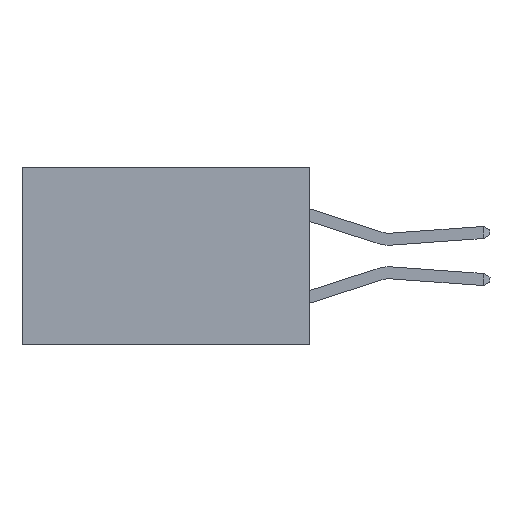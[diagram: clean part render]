
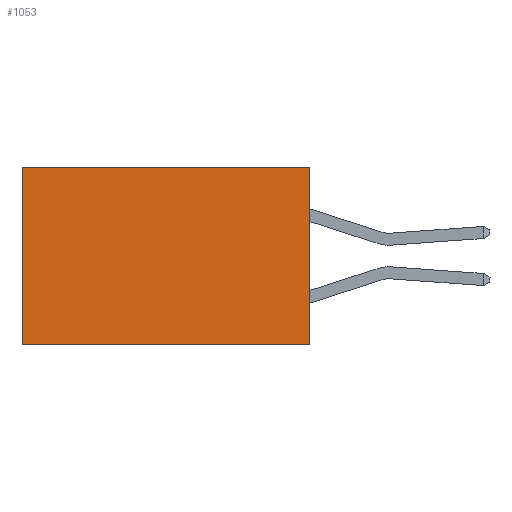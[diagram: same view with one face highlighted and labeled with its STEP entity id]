
A CAD part, left-side view. The second image highlights one B-rep face of the part: STEP entity #1053.
In plain terms, the highlighted planar face has unit normal (-1, 0, 0).
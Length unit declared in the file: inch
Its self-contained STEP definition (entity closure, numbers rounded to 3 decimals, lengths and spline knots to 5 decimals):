
#210 = EDGE_CURVE ( 'NONE', #5877, #9715, #4366, .T. ) ;
#818 = EDGE_CURVE ( 'NONE', #899, #9715, #8871, .T. ) ;
#899 = VERTEX_POINT ( 'NONE', #14866 ) ;
#1053 = ADVANCED_FACE ( 'NONE', ( #9055 ), #14499, .F. ) ;
#1126 = VECTOR ( 'NONE', #7966, 39.37008 ) ;
#1399 = CARTESIAN_POINT ( 'NONE',  ( 0.298, 0.6, 0. ) ) ;
#1630 = DIRECTION ( 'NONE',  ( 1., 0., 0. ) ) ;
#1676 = CARTESIAN_POINT ( 'NONE',  ( 0.298, 0., -0.37 ) ) ;
#1887 = CARTESIAN_POINT ( 'NONE',  ( 0.298, 0., 0. ) ) ;
#2750 = VECTOR ( 'NONE', #5408, 39.37008 ) ;
#3224 = ORIENTED_EDGE ( 'NONE', *, *, #13820, .F. ) ;
#3699 = CARTESIAN_POINT ( 'NONE',  ( 0.298, 0., 0. ) ) ;
#4366 = LINE ( 'NONE', #6325, #7005 ) ;
#4699 = VERTEX_POINT ( 'NONE', #11175 ) ;
#5408 = DIRECTION ( 'NONE',  ( 0., 0., -1. ) ) ;
#5877 = VERTEX_POINT ( 'NONE', #1676 ) ;
#6214 = AXIS2_PLACEMENT_3D ( 'NONE', #3699, #1630, #10070 ) ;
#6271 = DIRECTION ( 'NONE',  ( 0., 0., -1. ) ) ;
#6325 = CARTESIAN_POINT ( 'NONE',  ( 0.298, 0., -0.37 ) ) ;
#7005 = VECTOR ( 'NONE', #7495, 39.37008 ) ;
#7204 = ORIENTED_EDGE ( 'NONE', *, *, #12175, .T. ) ;
#7495 = DIRECTION ( 'NONE',  ( 0., 1., 0. ) ) ;
#7966 = DIRECTION ( 'NONE',  ( 0., 1., 0. ) ) ;
#8634 = LINE ( 'NONE', #13759, #2750 ) ;
#8871 = LINE ( 'NONE', #1399, #14891 ) ;
#9055 = FACE_OUTER_BOUND ( 'NONE', #9122, .T. ) ;
#9122 = EDGE_LOOP ( 'NONE', ( #9855, #10614, #3224, #7204 ) ) ;
#9715 = VERTEX_POINT ( 'NONE', #10079 ) ;
#9855 = ORIENTED_EDGE ( 'NONE', *, *, #818, .T. ) ;
#10070 = DIRECTION ( 'NONE',  ( 0., 0., -1. ) ) ;
#10079 = CARTESIAN_POINT ( 'NONE',  ( 0.298, 0.6, -0.37 ) ) ;
#10614 = ORIENTED_EDGE ( 'NONE', *, *, #210, .F. ) ;
#10928 = LINE ( 'NONE', #1887, #1126 ) ;
#11175 = CARTESIAN_POINT ( 'NONE',  ( 0.298, 0., 0. ) ) ;
#12175 = EDGE_CURVE ( 'NONE', #4699, #899, #10928, .T. ) ;
#13759 = CARTESIAN_POINT ( 'NONE',  ( 0.298, 0., 0. ) ) ;
#13820 = EDGE_CURVE ( 'NONE', #4699, #5877, #8634, .T. ) ;
#14499 = PLANE ( 'NONE',  #6214 ) ;
#14866 = CARTESIAN_POINT ( 'NONE',  ( 0.298, 0.6, 0. ) ) ;
#14891 = VECTOR ( 'NONE', #6271, 39.37008 ) ;
